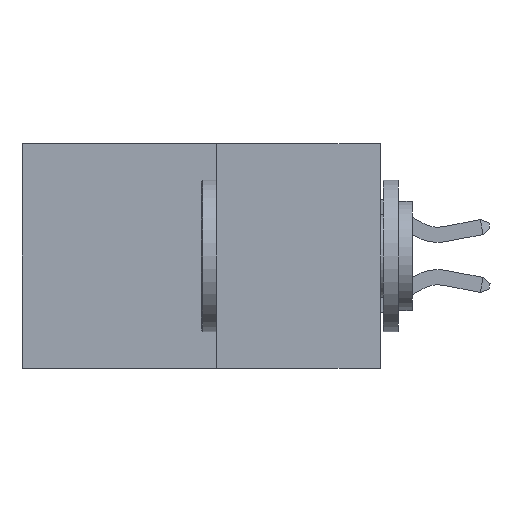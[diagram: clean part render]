
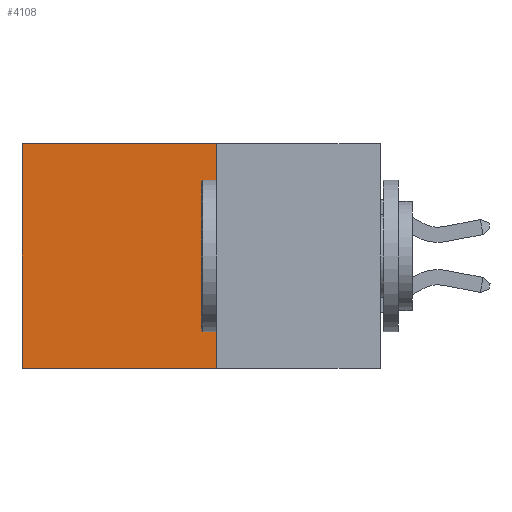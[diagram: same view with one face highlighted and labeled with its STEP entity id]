
A CAD part, left-side view. The second image highlights one B-rep face of the part: STEP entity #4108.
In plain terms, the highlighted planar face has unit normal (-1, 0, 0).
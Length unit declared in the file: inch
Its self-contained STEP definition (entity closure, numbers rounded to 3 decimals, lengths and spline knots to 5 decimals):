
#394 = EDGE_CURVE ( 'NONE', #1967, #4135, #5543, .T. ) ;
#1033 = DIRECTION ( 'NONE',  ( 0., 0., -1. ) ) ;
#1598 = LINE ( 'NONE', #5556, #5469 ) ;
#1967 = VERTEX_POINT ( 'NONE', #4015 ) ;
#2912 = AXIS2_PLACEMENT_3D ( 'NONE', #8753, #8688, #8686 ) ;
#3534 = VECTOR ( 'NONE', #5682, 39.37008 ) ;
#3610 = ORIENTED_EDGE ( 'NONE', *, *, #9393, .T. ) ;
#3835 = ORIENTED_EDGE ( 'NONE', *, *, #8428, .F. ) ;
#4015 = CARTESIAN_POINT ( 'NONE',  ( 0.277, 0.27, 0. ) ) ;
#4038 = DIRECTION ( 'NONE',  ( 0., 1., 0. ) ) ;
#4108 = ADVANCED_FACE ( 'NONE', ( #8926 ), #8720, .F. ) ;
#4135 = VERTEX_POINT ( 'NONE', #8652 ) ;
#4699 = DIRECTION ( 'NONE',  ( 0., 0., -1. ) ) ;
#4860 = VERTEX_POINT ( 'NONE', #4885 ) ;
#4885 = CARTESIAN_POINT ( 'NONE',  ( 0.277, 0.59, -0.37 ) ) ;
#5125 = EDGE_LOOP ( 'NONE', ( #3610, #3835, #5848, #9684 ) ) ;
#5390 = VECTOR ( 'NONE', #4699, 39.37008 ) ;
#5469 = VECTOR ( 'NONE', #4038, 39.37008 ) ;
#5543 = LINE ( 'NONE', #7781, #3534 ) ;
#5556 = CARTESIAN_POINT ( 'NONE',  ( 0.277, 0.27, -0.37 ) ) ;
#5625 = LINE ( 'NONE', #9100, #5390 ) ;
#5682 = DIRECTION ( 'NONE',  ( 0., 1., 0. ) ) ;
#5848 = ORIENTED_EDGE ( 'NONE', *, *, #6453, .F. ) ;
#6398 = CARTESIAN_POINT ( 'NONE',  ( 0.277, 0.59, -0.37 ) ) ;
#6453 = EDGE_CURVE ( 'NONE', #1967, #8469, #5625, .T. ) ;
#7067 = CARTESIAN_POINT ( 'NONE',  ( 0.277, 0.27, -0.37 ) ) ;
#7781 = CARTESIAN_POINT ( 'NONE',  ( 0.277, 0.27, 0. ) ) ;
#8201 = LINE ( 'NONE', #6398, #9641 ) ;
#8428 = EDGE_CURVE ( 'NONE', #8469, #4860, #1598, .T. ) ;
#8469 = VERTEX_POINT ( 'NONE', #7067 ) ;
#8652 = CARTESIAN_POINT ( 'NONE',  ( 0.277, 0.59, 0. ) ) ;
#8686 = DIRECTION ( 'NONE',  ( 0., 0., -1. ) ) ;
#8688 = DIRECTION ( 'NONE',  ( 1., 0., 0. ) ) ;
#8720 = PLANE ( 'NONE',  #2912 ) ;
#8753 = CARTESIAN_POINT ( 'NONE',  ( 0.277, 0.27, -0.37 ) ) ;
#8926 = FACE_OUTER_BOUND ( 'NONE', #5125, .T. ) ;
#9100 = CARTESIAN_POINT ( 'NONE',  ( 0.277, 0.27, -0.37 ) ) ;
#9393 = EDGE_CURVE ( 'NONE', #4135, #4860, #8201, .T. ) ;
#9641 = VECTOR ( 'NONE', #1033, 39.37008 ) ;
#9684 = ORIENTED_EDGE ( 'NONE', *, *, #394, .T. ) ;
